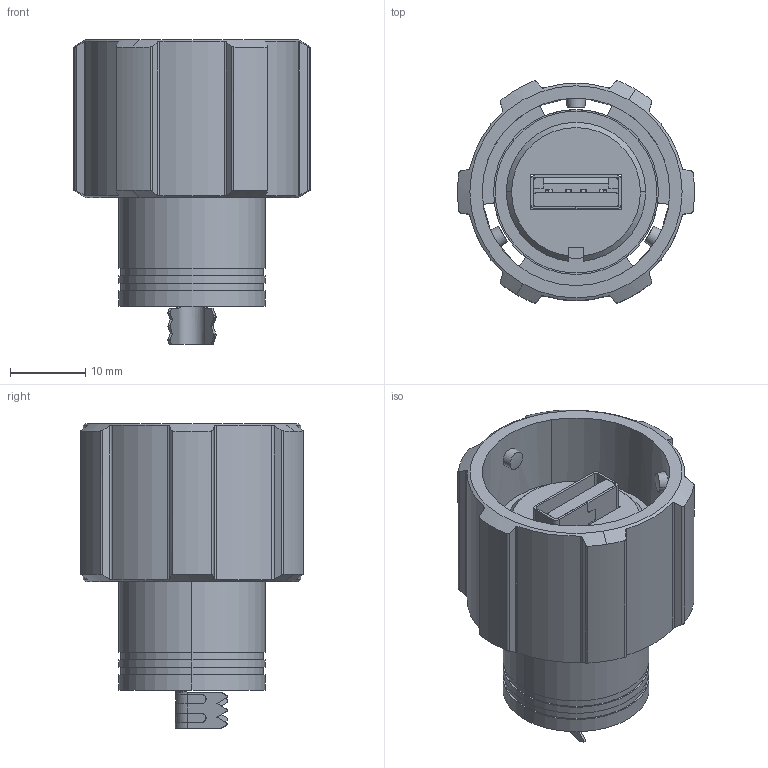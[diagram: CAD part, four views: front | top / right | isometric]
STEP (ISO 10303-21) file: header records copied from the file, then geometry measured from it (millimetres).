
FILE_DESCRIPTION (( 'STEP AP214' ), '1' );
FILE_NAME ('690-W04-260-013.STEP', '2021-04-12T16:33:46', ( '' ), ( '' ), 'SwSTEP 2.0', 'SolidWorks 2020', '' );
FILE_SCHEMA (( 'AUTOMOTIVE_DESIGN' ));
Length unit declared in the file: millimetre
Products named in the file (10): USB CONTACT ASSY 690-W04-X60-013; SHELL2 690-W04-X60-013; SHELL1 690-W04-X60-013; USB CONTACT HOUSING 690-W04-X60-013; CONTACTS 690-W04-X60-013; 690-W04-260-013; O-RING 690-W04-X60-013; HOUSING INNER  690-W04-X60-013; HOUSING OUTER  690-W04-X60-013; USB ASSY 690-W04-X60-013
Assembly tree (9 placements, depth 4):
  690-W04-260-013
    USB ASSY 690-W04-X60-013
      USB CONTACT ASSY 690-W04-X60-013
        USB CONTACT HOUSING 690-W04-X60-013
        CONTACTS 690-W04-X60-013
      SHELL1 690-W04-X60-013
      SHELL2 690-W04-X60-013
    HOUSING INNER  690-W04-X60-013
    O-RING 690-W04-X60-013
    HOUSING OUTER  690-W04-X60-013
Bounding box: 31.45 x 29.5 x 40.51 mm (x, y, z)
Volume: 10059.6 mm3; surface area: 12994.9 mm2
Topology: 10 solids, 10 shells, 980 faces, 2806 edges, 1840 vertices
Faces by surface type: plane 670, cylinder 282, bspline 19, cone 9
Entity records: 34182 total; most frequent: CARTESIAN_POINT 8701, ORIENTED_EDGE 5612, DIRECTION 4698, EDGE_CURVE 2806, LINE 2038, VECTOR 2038, VERTEX_POINT 1840, AXIS2_PLACEMENT_3D 1330
